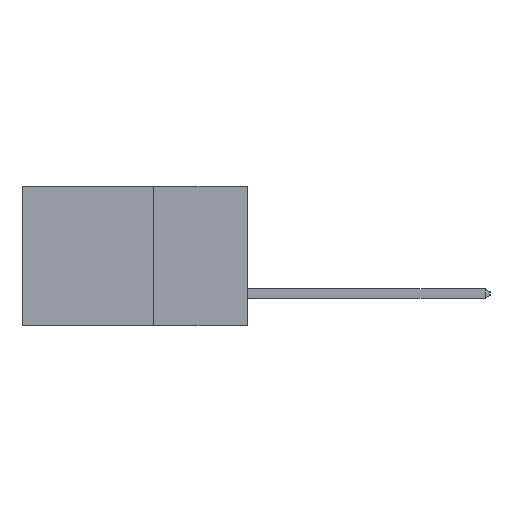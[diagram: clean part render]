
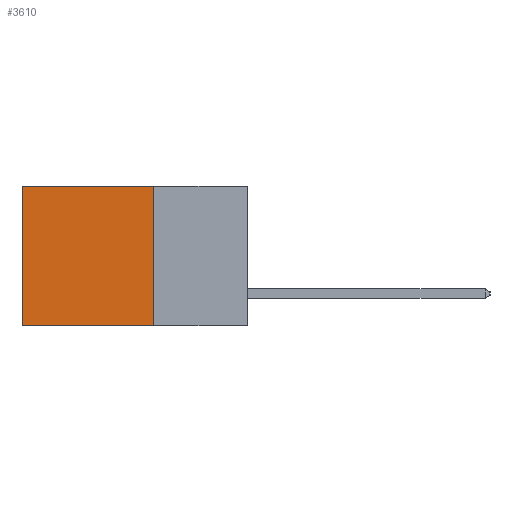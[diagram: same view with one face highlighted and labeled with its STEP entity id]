
A CAD part, left-side view. The second image highlights one B-rep face of the part: STEP entity #3610.
In plain terms, the highlighted planar face has unit normal (-1, 0, 0).
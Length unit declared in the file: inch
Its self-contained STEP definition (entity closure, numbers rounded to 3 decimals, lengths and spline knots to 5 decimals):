
#928 = LINE ( 'NONE', #6447, #3590 ) ;
#998 = ORIENTED_EDGE ( 'NONE', *, *, #2345, .T. ) ;
#1472 = VERTEX_POINT ( 'NONE', #4057 ) ;
#1584 = VERTEX_POINT ( 'NONE', #10883 ) ;
#1692 = CARTESIAN_POINT ( 'NONE',  ( 0.2615, 0.25, -0.37 ) ) ;
#1701 = DIRECTION ( 'NONE',  ( 0., 1., 0. ) ) ;
#1845 = VECTOR ( 'NONE', #10564, 39.37008 ) ;
#2345 = EDGE_CURVE ( 'NONE', #11172, #4109, #9604, .T. ) ;
#2892 = CARTESIAN_POINT ( 'NONE',  ( 0.2615, 0.6, 0. ) ) ;
#3590 = VECTOR ( 'NONE', #1701, 39.37008 ) ;
#3610 = ADVANCED_FACE ( 'NONE', ( #10087 ), #7187, .F. ) ;
#3662 = DIRECTION ( 'NONE',  ( 0., 0., -1. ) ) ;
#3956 = ORIENTED_EDGE ( 'NONE', *, *, #7685, .F. ) ;
#4057 = CARTESIAN_POINT ( 'NONE',  ( 0.2615, 0.25, 0. ) ) ;
#4109 = VERTEX_POINT ( 'NONE', #6350 ) ;
#4468 = LINE ( 'NONE', #8928, #1845 ) ;
#4538 = EDGE_CURVE ( 'NONE', #1584, #4109, #928, .T. ) ;
#5665 = EDGE_CURVE ( 'NONE', #1472, #11172, #4468, .T. ) ;
#5831 = CARTESIAN_POINT ( 'NONE',  ( 0.2615, 0.6, -0.37 ) ) ;
#6350 = CARTESIAN_POINT ( 'NONE',  ( 0.2615, 0.6, -0.37 ) ) ;
#6447 = CARTESIAN_POINT ( 'NONE',  ( 0.2615, 0.25, -0.37 ) ) ;
#7125 = EDGE_LOOP ( 'NONE', ( #998, #10637, #3956, #10878 ) ) ;
#7187 = PLANE ( 'NONE',  #10447 ) ;
#7685 = EDGE_CURVE ( 'NONE', #1472, #1584, #9121, .T. ) ;
#8214 = DIRECTION ( 'NONE',  ( 0., 0., -1. ) ) ;
#8322 = CARTESIAN_POINT ( 'NONE',  ( 0.2615, 0.25, -0.37 ) ) ;
#8928 = CARTESIAN_POINT ( 'NONE',  ( 0.2615, 0.25, 0. ) ) ;
#9121 = LINE ( 'NONE', #1692, #9374 ) ;
#9272 = VECTOR ( 'NONE', #3662, 39.37008 ) ;
#9374 = VECTOR ( 'NONE', #8214, 39.37008 ) ;
#9604 = LINE ( 'NONE', #5831, #9272 ) ;
#10087 = FACE_OUTER_BOUND ( 'NONE', #7125, .T. ) ;
#10447 = AXIS2_PLACEMENT_3D ( 'NONE', #8322, #10750, #11023 ) ;
#10564 = DIRECTION ( 'NONE',  ( 0., 1., 0. ) ) ;
#10637 = ORIENTED_EDGE ( 'NONE', *, *, #4538, .F. ) ;
#10750 = DIRECTION ( 'NONE',  ( 1., 0., 0. ) ) ;
#10878 = ORIENTED_EDGE ( 'NONE', *, *, #5665, .T. ) ;
#10883 = CARTESIAN_POINT ( 'NONE',  ( 0.2615, 0.25, -0.37 ) ) ;
#11023 = DIRECTION ( 'NONE',  ( 0., 0., -1. ) ) ;
#11172 = VERTEX_POINT ( 'NONE', #2892 ) ;
